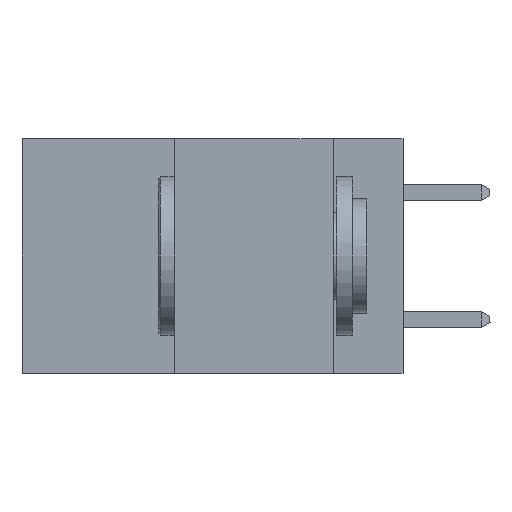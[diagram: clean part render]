
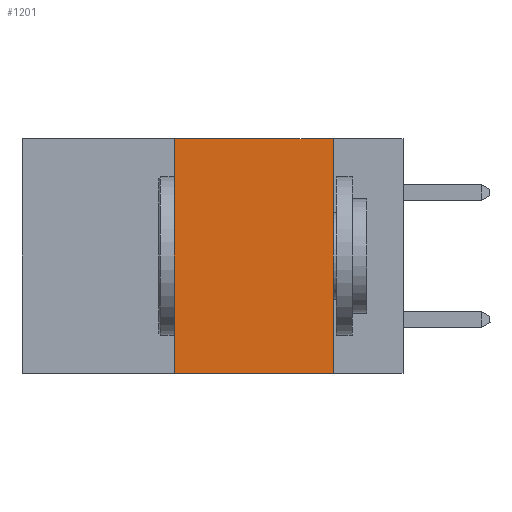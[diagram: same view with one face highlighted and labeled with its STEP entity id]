
A CAD part, left-side view. The second image highlights one B-rep face of the part: STEP entity #1201.
In plain terms, the highlighted planar face has unit normal (-1, 0, 0).
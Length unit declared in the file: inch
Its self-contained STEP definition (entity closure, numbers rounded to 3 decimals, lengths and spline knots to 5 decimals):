
#127 = LINE ( 'NONE', #18235, #13483 ) ;
#758 = VERTEX_POINT ( 'NONE', #18580 ) ;
#1201 = ADVANCED_FACE ( 'NONE', ( #2569 ), #8527, .F. ) ;
#2450 = VECTOR ( 'NONE', #15280, 39.37008 ) ;
#2569 = FACE_OUTER_BOUND ( 'NONE', #8915, .T. ) ;
#2948 = ORIENTED_EDGE ( 'NONE', *, *, #21006, .F. ) ;
#4370 = DIRECTION ( 'NONE',  ( 0., -1., 0. ) ) ;
#5378 = CARTESIAN_POINT ( 'NONE',  ( 0., 0.11, 0. ) ) ;
#6189 = VECTOR ( 'NONE', #12738, 39.37008 ) ;
#7662 = VECTOR ( 'NONE', #14057, 39.37008 ) ;
#7721 = EDGE_CURVE ( 'NONE', #21366, #8561, #20068, .T. ) ;
#8371 = DIRECTION ( 'NONE',  ( 0., 0., -1. ) ) ;
#8449 = DIRECTION ( 'NONE',  ( 1., 0., 0. ) ) ;
#8476 = CARTESIAN_POINT ( 'NONE',  ( 0., 0.6, 0. ) ) ;
#8527 = PLANE ( 'NONE',  #17823 ) ;
#8561 = VERTEX_POINT ( 'NONE', #20246 ) ;
#8915 = EDGE_LOOP ( 'NONE', ( #2948, #12726, #17880, #13778 ) ) ;
#11099 = CARTESIAN_POINT ( 'NONE',  ( 0., 0.6, -0.37 ) ) ;
#12726 = ORIENTED_EDGE ( 'NONE', *, *, #16752, .F. ) ;
#12738 = DIRECTION ( 'NONE',  ( 0., -1., 0. ) ) ;
#13483 = VECTOR ( 'NONE', #4370, 39.37008 ) ;
#13778 = ORIENTED_EDGE ( 'NONE', *, *, #7721, .T. ) ;
#14057 = DIRECTION ( 'NONE',  ( 0., 0., -1. ) ) ;
#15280 = DIRECTION ( 'NONE',  ( 0., 0., 1. ) ) ;
#15363 = EDGE_CURVE ( 'NONE', #21366, #758, #16268, .T. ) ;
#16268 = LINE ( 'NONE', #22240, #2450 ) ;
#16411 = VERTEX_POINT ( 'NONE', #22585 ) ;
#16752 = EDGE_CURVE ( 'NONE', #758, #16411, #127, .T. ) ;
#17823 = AXIS2_PLACEMENT_3D ( 'NONE', #8476, #8449, #8371 ) ;
#17880 = ORIENTED_EDGE ( 'NONE', *, *, #15363, .F. ) ;
#18235 = CARTESIAN_POINT ( 'NONE',  ( 0., 0.6, 0. ) ) ;
#18580 = CARTESIAN_POINT ( 'NONE',  ( 0., 0.36, 0. ) ) ;
#20068 = LINE ( 'NONE', #11099, #6189 ) ;
#20180 = CARTESIAN_POINT ( 'NONE',  ( 0., 0.36, -0.37 ) ) ;
#20246 = CARTESIAN_POINT ( 'NONE',  ( 0., 0.11, -0.37 ) ) ;
#21006 = EDGE_CURVE ( 'NONE', #16411, #8561, #21541, .T. ) ;
#21366 = VERTEX_POINT ( 'NONE', #20180 ) ;
#21541 = LINE ( 'NONE', #5378, #7662 ) ;
#22240 = CARTESIAN_POINT ( 'NONE',  ( 0., 0.36, 0. ) ) ;
#22585 = CARTESIAN_POINT ( 'NONE',  ( 0., 0.11, 0. ) ) ;
